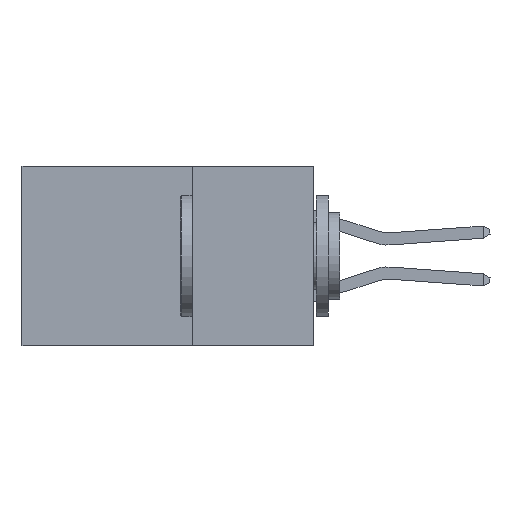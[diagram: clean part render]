
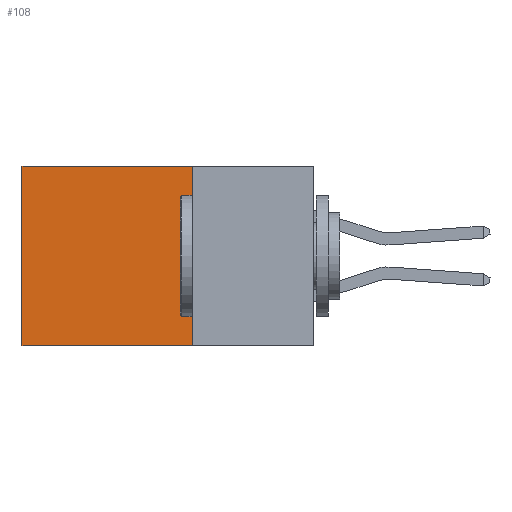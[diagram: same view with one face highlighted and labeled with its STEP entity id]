
A CAD part, left-side view. The second image highlights one B-rep face of the part: STEP entity #108.
In plain terms, the highlighted planar face has unit normal (-1, 0, 0).
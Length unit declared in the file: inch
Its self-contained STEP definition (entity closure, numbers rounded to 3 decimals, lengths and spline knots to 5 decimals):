
#108 = ADVANCED_FACE ( 'NONE', ( #6813 ), #21058, .F. ) ;
#1334 = LINE ( 'NONE', #9906, #18264 ) ;
#1780 = CARTESIAN_POINT ( 'NONE',  ( 0.2875, 0.25, 0. ) ) ;
#3944 = VECTOR ( 'NONE', #6384, 39.37008 ) ;
#4555 = VERTEX_POINT ( 'NONE', #16008 ) ;
#4885 = DIRECTION ( 'NONE',  ( 1., 0., 0. ) ) ;
#4974 = CARTESIAN_POINT ( 'NONE',  ( 0.2875, 0.6, 0. ) ) ;
#5139 = DIRECTION ( 'NONE',  ( 0., 0., -1. ) ) ;
#5386 = ORIENTED_EDGE ( 'NONE', *, *, #18028, .F. ) ;
#6103 = EDGE_CURVE ( 'NONE', #12017, #7373, #14563, .T. ) ;
#6384 = DIRECTION ( 'NONE',  ( 0., 0., -1. ) ) ;
#6616 = EDGE_CURVE ( 'NONE', #4555, #7373, #11481, .T. ) ;
#6716 = CARTESIAN_POINT ( 'NONE',  ( 0.2875, 0.25, 0. ) ) ;
#6813 = FACE_OUTER_BOUND ( 'NONE', #15535, .T. ) ;
#7373 = VERTEX_POINT ( 'NONE', #17706 ) ;
#7871 = ORIENTED_EDGE ( 'NONE', *, *, #6616, .T. ) ;
#8290 = DIRECTION ( 'NONE',  ( 0., 0., -1. ) ) ;
#9267 = CARTESIAN_POINT ( 'NONE',  ( 0.2875, 0.25, -0.37 ) ) ;
#9676 = DIRECTION ( 'NONE',  ( 0., 1., 0. ) ) ;
#9906 = CARTESIAN_POINT ( 'NONE',  ( 0.2875, 0.25, 0. ) ) ;
#10324 = CARTESIAN_POINT ( 'NONE',  ( 0.2875, 0.25, 0. ) ) ;
#11294 = LINE ( 'NONE', #10324, #3944 ) ;
#11481 = LINE ( 'NONE', #4974, #17673 ) ;
#11785 = CARTESIAN_POINT ( 'NONE',  ( 0.2875, 0.25, -0.37 ) ) ;
#12017 = VERTEX_POINT ( 'NONE', #11785 ) ;
#13089 = EDGE_CURVE ( 'NONE', #13609, #4555, #1334, .T. ) ;
#13224 = ORIENTED_EDGE ( 'NONE', *, *, #13089, .T. ) ;
#13609 = VERTEX_POINT ( 'NONE', #1780 ) ;
#14563 = LINE ( 'NONE', #9267, #22975 ) ;
#15535 = EDGE_LOOP ( 'NONE', ( #7871, #16253, #5386, #13224 ) ) ;
#16008 = CARTESIAN_POINT ( 'NONE',  ( 0.2875, 0.6, 0. ) ) ;
#16253 = ORIENTED_EDGE ( 'NONE', *, *, #6103, .F. ) ;
#17673 = VECTOR ( 'NONE', #5139, 39.37008 ) ;
#17706 = CARTESIAN_POINT ( 'NONE',  ( 0.2875, 0.6, -0.37 ) ) ;
#18028 = EDGE_CURVE ( 'NONE', #13609, #12017, #11294, .T. ) ;
#18264 = VECTOR ( 'NONE', #9676, 39.37008 ) ;
#19028 = AXIS2_PLACEMENT_3D ( 'NONE', #6716, #4885, #8290 ) ;
#21058 = PLANE ( 'NONE',  #19028 ) ;
#21776 = DIRECTION ( 'NONE',  ( 0., 1., 0. ) ) ;
#22975 = VECTOR ( 'NONE', #21776, 39.37008 ) ;
